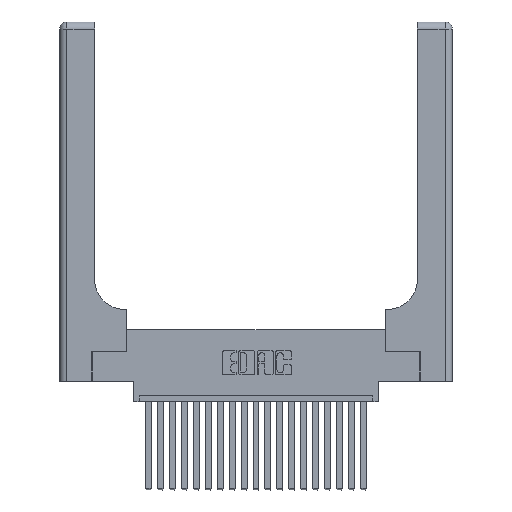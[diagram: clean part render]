
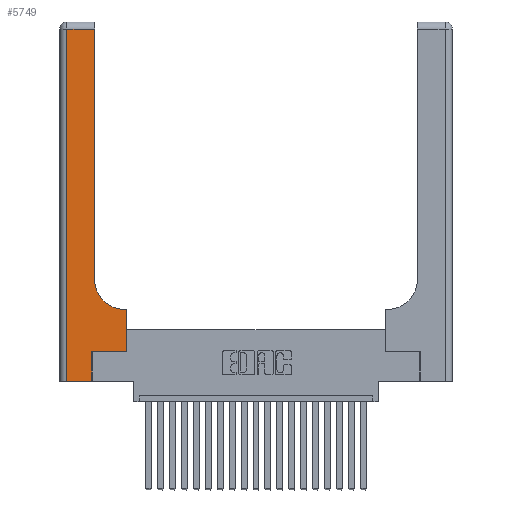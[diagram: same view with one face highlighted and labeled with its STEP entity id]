
A CAD part, top view. The second image highlights one B-rep face of the part: STEP entity #5749.
In plain terms, the highlighted planar face has unit normal (0, 0, 1).
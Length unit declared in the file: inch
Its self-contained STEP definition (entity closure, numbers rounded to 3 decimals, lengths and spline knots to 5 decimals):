
#156 = CARTESIAN_POINT ( 'NONE',  ( 0.06, 3., 0.37 ) ) ;
#275 = ORIENTED_EDGE ( 'NONE', *, *, #16148, .T. ) ;
#1137 = DIRECTION ( 'NONE',  ( 0., 0., -1. ) ) ;
#1869 = CIRCLE ( 'NONE', #6989, 0.25 ) ;
#2172 = DIRECTION ( 'NONE',  ( 1., 0., 0. ) ) ;
#2297 = VECTOR ( 'NONE', #3233, 39.37008 ) ;
#2438 = VERTEX_POINT ( 'NONE', #20832 ) ;
#2477 = ORIENTED_EDGE ( 'NONE', *, *, #5474, .T. ) ;
#2492 = ORIENTED_EDGE ( 'NONE', *, *, #10700, .T. ) ;
#2548 = DIRECTION ( 'NONE',  ( 0., 1., 0. ) ) ;
#2875 = ORIENTED_EDGE ( 'NONE', *, *, #15985, .T. ) ;
#3233 = DIRECTION ( 'NONE',  ( 0., 1., 0. ) ) ;
#3475 = VECTOR ( 'NONE', #5928, 39.37008 ) ;
#3498 = VECTOR ( 'NONE', #13218, 39.37008 ) ;
#3580 = CARTESIAN_POINT ( 'NONE',  ( 0.5585, 0.25, 0.37 ) ) ;
#4173 = VERTEX_POINT ( 'NONE', #14651 ) ;
#4978 = EDGE_CURVE ( 'NONE', #13999, #2438, #20012, .T. ) ;
#5238 = DIRECTION ( 'NONE',  ( 0., -1., 0. ) ) ;
#5474 = EDGE_CURVE ( 'NONE', #4173, #10082, #18636, .T. ) ;
#5749 = ADVANCED_FACE ( 'NONE', ( #8844 ), #5983, .F. ) ;
#5928 = DIRECTION ( 'NONE',  ( -1., 0., 0. ) ) ;
#5983 = PLANE ( 'NONE',  #14670 ) ;
#6183 = ORIENTED_EDGE ( 'NONE', *, *, #22002, .T. ) ;
#6894 = VERTEX_POINT ( 'NONE', #16625 ) ;
#6989 = AXIS2_PLACEMENT_3D ( 'NONE', #12387, #17850, #7361 ) ;
#7277 = CARTESIAN_POINT ( 'NONE',  ( 0., 0., 0.37 ) ) ;
#7361 = DIRECTION ( 'NONE',  ( 1., 0., 0. ) ) ;
#7551 = LINE ( 'NONE', #156, #9199 ) ;
#7691 = EDGE_CURVE ( 'NONE', #15483, #4173, #10918, .T. ) ;
#8127 = LINE ( 'NONE', #21404, #3475 ) ;
#8311 = CARTESIAN_POINT ( 'NONE',  ( 0.269, 0.25, 0.37 ) ) ;
#8468 = ORIENTED_EDGE ( 'NONE', *, *, #7691, .T. ) ;
#8683 = LINE ( 'NONE', #21540, #22247 ) ;
#8844 = FACE_OUTER_BOUND ( 'NONE', #18328, .T. ) ;
#9199 = VECTOR ( 'NONE', #5238, 39.37008 ) ;
#9970 = CARTESIAN_POINT ( 'NONE',  ( 0.06, 0., 0.37 ) ) ;
#10082 = VERTEX_POINT ( 'NONE', #8311 ) ;
#10229 = CARTESIAN_POINT ( 'NONE',  ( 0.269, 0., 0.37 ) ) ;
#10700 = EDGE_CURVE ( 'NONE', #6894, #15936, #1869, .T. ) ;
#10720 = CARTESIAN_POINT ( 'NONE',  ( 0.5585, 0.25, 0.37 ) ) ;
#10868 = LINE ( 'NONE', #18464, #3498 ) ;
#10918 = LINE ( 'NONE', #7277, #13890 ) ;
#11120 = CARTESIAN_POINT ( 'NONE',  ( 0.2915, 0.85, 0.37 ) ) ;
#11728 = EDGE_CURVE ( 'NONE', #2438, #6894, #8127, .T. ) ;
#12024 = EDGE_CURVE ( 'NONE', #14013, #15483, #7551, .T. ) ;
#12355 = DIRECTION ( 'NONE',  ( 0., 1., 0. ) ) ;
#12387 = CARTESIAN_POINT ( 'NONE',  ( 0.5415, 0.85, 0.37 ) ) ;
#12547 = CARTESIAN_POINT ( 'NONE',  ( 0.269, 0.25, 0.37 ) ) ;
#13218 = DIRECTION ( 'NONE',  ( -1., 0., 0. ) ) ;
#13890 = VECTOR ( 'NONE', #14988, 39.37008 ) ;
#13953 = ORIENTED_EDGE ( 'NONE', *, *, #12024, .T. ) ;
#13999 = VERTEX_POINT ( 'NONE', #10720 ) ;
#14013 = VERTEX_POINT ( 'NONE', #21229 ) ;
#14651 = CARTESIAN_POINT ( 'NONE',  ( 0.269, 0., 0.37 ) ) ;
#14670 = AXIS2_PLACEMENT_3D ( 'NONE', #21799, #1137, #19936 ) ;
#14988 = DIRECTION ( 'NONE',  ( 1., 0., 0. ) ) ;
#15483 = VERTEX_POINT ( 'NONE', #9970 ) ;
#15911 = VERTEX_POINT ( 'NONE', #19744 ) ;
#15936 = VERTEX_POINT ( 'NONE', #11120 ) ;
#15985 = EDGE_CURVE ( 'NONE', #15936, #15911, #8683, .T. ) ;
#16148 = EDGE_CURVE ( 'NONE', #15911, #14013, #10868, .T. ) ;
#16625 = CARTESIAN_POINT ( 'NONE',  ( 0.5415, 0.6, 0.37 ) ) ;
#17042 = ORIENTED_EDGE ( 'NONE', *, *, #11728, .T. ) ;
#17667 = LINE ( 'NONE', #12547, #18242 ) ;
#17850 = DIRECTION ( 'NONE',  ( 0., 0., -1. ) ) ;
#18242 = VECTOR ( 'NONE', #2172, 39.37008 ) ;
#18328 = EDGE_LOOP ( 'NONE', ( #2875, #275, #13953, #8468, #2477, #6183, #21259, #17042, #2492 ) ) ;
#18396 = VECTOR ( 'NONE', #12355, 39.37008 ) ;
#18464 = CARTESIAN_POINT ( 'NONE',  ( 0., 2.94, 0.37 ) ) ;
#18636 = LINE ( 'NONE', #10229, #2297 ) ;
#19744 = CARTESIAN_POINT ( 'NONE',  ( 0.2915, 2.94, 0.37 ) ) ;
#19936 = DIRECTION ( 'NONE',  ( -1., 0., 0. ) ) ;
#20012 = LINE ( 'NONE', #3580, #18396 ) ;
#20832 = CARTESIAN_POINT ( 'NONE',  ( 0.5585, 0.6, 0.37 ) ) ;
#21229 = CARTESIAN_POINT ( 'NONE',  ( 0.06, 2.94, 0.37 ) ) ;
#21259 = ORIENTED_EDGE ( 'NONE', *, *, #4978, .T. ) ;
#21404 = CARTESIAN_POINT ( 'NONE',  ( 0.2915, 0.6, 0.37 ) ) ;
#21540 = CARTESIAN_POINT ( 'NONE',  ( 0.2915, 3., 0.37 ) ) ;
#21799 = CARTESIAN_POINT ( 'NONE',  ( 0., 3., 0.37 ) ) ;
#22002 = EDGE_CURVE ( 'NONE', #10082, #13999, #17667, .T. ) ;
#22247 = VECTOR ( 'NONE', #2548, 39.37008 ) ;
